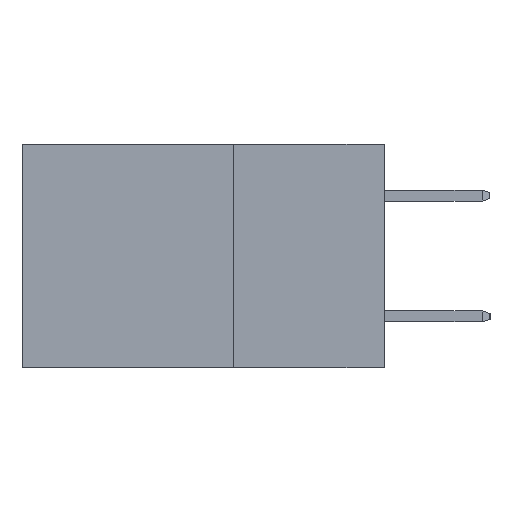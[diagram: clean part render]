
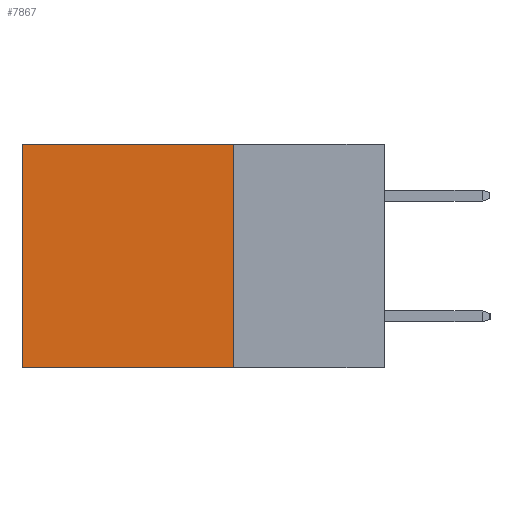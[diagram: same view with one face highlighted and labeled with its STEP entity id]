
A CAD part, left-side view. The second image highlights one B-rep face of the part: STEP entity #7867.
In plain terms, the highlighted planar face has unit normal (-1, 0, 0).
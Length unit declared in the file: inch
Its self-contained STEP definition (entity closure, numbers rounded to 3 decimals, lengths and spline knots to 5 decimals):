
#585 = VECTOR ( 'NONE', #9636, 39.37008 ) ;
#660 = EDGE_CURVE ( 'NONE', #4502, #2558, #2930, .T. ) ;
#825 = CARTESIAN_POINT ( 'NONE',  ( 0.2615, 0.25, -0.37 ) ) ;
#1357 = LINE ( 'NONE', #825, #585 ) ;
#1524 = ORIENTED_EDGE ( 'NONE', *, *, #660, .F. ) ;
#1853 = CARTESIAN_POINT ( 'NONE',  ( 0.2615, 0.25, 0. ) ) ;
#2021 = AXIS2_PLACEMENT_3D ( 'NONE', #2607, #3444, #8974 ) ;
#2558 = VERTEX_POINT ( 'NONE', #5879 ) ;
#2607 = CARTESIAN_POINT ( 'NONE',  ( 0.2615, 0.25, -0.37 ) ) ;
#2653 = DIRECTION ( 'NONE',  ( 0., 0., -1. ) ) ;
#2666 = VECTOR ( 'NONE', #2653, 39.37008 ) ;
#2930 = LINE ( 'NONE', #5950, #2666 ) ;
#3444 = DIRECTION ( 'NONE',  ( 1., 0., 0. ) ) ;
#3472 = ORIENTED_EDGE ( 'NONE', *, *, #9699, .F. ) ;
#3747 = ORIENTED_EDGE ( 'NONE', *, *, #7199, .T. ) ;
#3979 = EDGE_CURVE ( 'NONE', #8521, #7284, #5045, .T. ) ;
#4138 = CARTESIAN_POINT ( 'NONE',  ( 0.2615, 0.6, -0.37 ) ) ;
#4154 = EDGE_LOOP ( 'NONE', ( #7483, #3472, #1524, #3747 ) ) ;
#4179 = DIRECTION ( 'NONE',  ( 0., 0., -1. ) ) ;
#4244 = VECTOR ( 'NONE', #7482, 39.37008 ) ;
#4502 = VERTEX_POINT ( 'NONE', #1853 ) ;
#5045 = LINE ( 'NONE', #4138, #9185 ) ;
#5123 = CARTESIAN_POINT ( 'NONE',  ( 0.2615, 0.25, 0. ) ) ;
#5220 = CARTESIAN_POINT ( 'NONE',  ( 0.2615, 0.6, -0.37 ) ) ;
#5879 = CARTESIAN_POINT ( 'NONE',  ( 0.2615, 0.25, -0.37 ) ) ;
#5950 = CARTESIAN_POINT ( 'NONE',  ( 0.2615, 0.25, -0.37 ) ) ;
#7199 = EDGE_CURVE ( 'NONE', #4502, #8521, #7955, .T. ) ;
#7284 = VERTEX_POINT ( 'NONE', #5220 ) ;
#7482 = DIRECTION ( 'NONE',  ( 0., 1., 0. ) ) ;
#7483 = ORIENTED_EDGE ( 'NONE', *, *, #3979, .T. ) ;
#7867 = ADVANCED_FACE ( 'NONE', ( #8549 ), #8208, .F. ) ;
#7955 = LINE ( 'NONE', #5123, #4244 ) ;
#8208 = PLANE ( 'NONE',  #2021 ) ;
#8521 = VERTEX_POINT ( 'NONE', #9725 ) ;
#8549 = FACE_OUTER_BOUND ( 'NONE', #4154, .T. ) ;
#8974 = DIRECTION ( 'NONE',  ( 0., 0., -1. ) ) ;
#9185 = VECTOR ( 'NONE', #4179, 39.37008 ) ;
#9636 = DIRECTION ( 'NONE',  ( 0., 1., 0. ) ) ;
#9699 = EDGE_CURVE ( 'NONE', #2558, #7284, #1357, .T. ) ;
#9725 = CARTESIAN_POINT ( 'NONE',  ( 0.2615, 0.6, 0. ) ) ;
